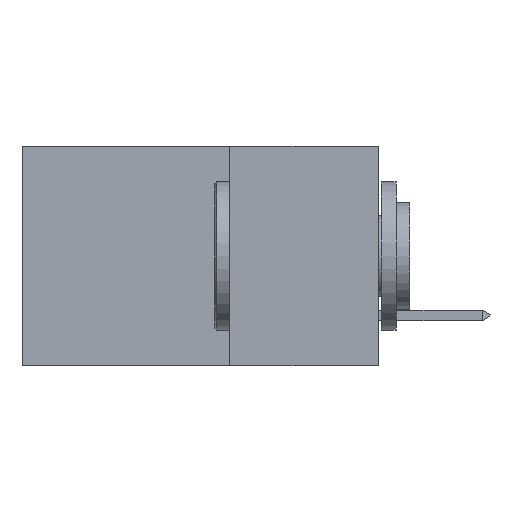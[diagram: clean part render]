
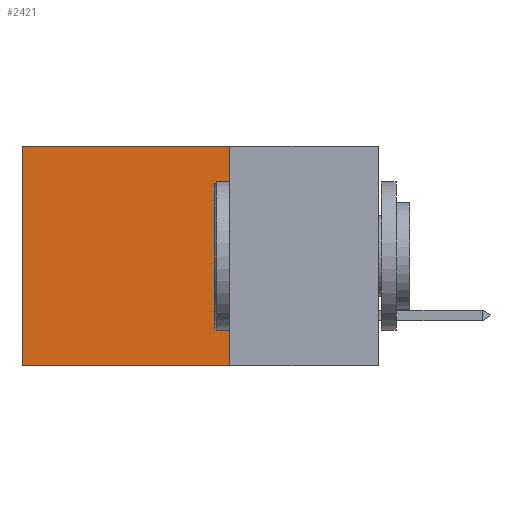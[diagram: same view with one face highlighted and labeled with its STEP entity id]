
A CAD part, left-side view. The second image highlights one B-rep face of the part: STEP entity #2421.
In plain terms, the highlighted planar face has unit normal (-1, 0, 0).
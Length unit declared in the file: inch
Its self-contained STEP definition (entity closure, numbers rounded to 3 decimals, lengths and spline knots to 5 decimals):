
#134 = CARTESIAN_POINT ( 'NONE',  ( 0.2615, 0.6, -0.37 ) ) ;
#1147 = VERTEX_POINT ( 'NONE', #4742 ) ;
#1373 = ORIENTED_EDGE ( 'NONE', *, *, #14383, .T. ) ;
#1987 = AXIS2_PLACEMENT_3D ( 'NONE', #10348, #13753, #13902 ) ;
#2421 = ADVANCED_FACE ( 'NONE', ( #10272 ), #9294, .F. ) ;
#2473 = EDGE_CURVE ( 'NONE', #3451, #9323, #14827, .T. ) ;
#2577 = CARTESIAN_POINT ( 'NONE',  ( 0.2615, 0.25, -0.37 ) ) ;
#2653 = LINE ( 'NONE', #2577, #9335 ) ;
#2990 = ORIENTED_EDGE ( 'NONE', *, *, #2473, .T. ) ;
#3451 = VERTEX_POINT ( 'NONE', #3565 ) ;
#3565 = CARTESIAN_POINT ( 'NONE',  ( 0.2615, 0.6, 0. ) ) ;
#4742 = CARTESIAN_POINT ( 'NONE',  ( 0.2615, 0.25, 0. ) ) ;
#4792 = DIRECTION ( 'NONE',  ( 0., 1., 0. ) ) ;
#5675 = CARTESIAN_POINT ( 'NONE',  ( 0.2615, 0.6, -0.37 ) ) ;
#5915 = LINE ( 'NONE', #13922, #9956 ) ;
#6710 = EDGE_LOOP ( 'NONE', ( #2990, #13027, #14347, #1373 ) ) ;
#6981 = LINE ( 'NONE', #12716, #7502 ) ;
#7502 = VECTOR ( 'NONE', #4792, 39.37008 ) ;
#7529 = VECTOR ( 'NONE', #12693, 39.37008 ) ;
#7780 = EDGE_CURVE ( 'NONE', #10533, #9323, #2653, .T. ) ;
#9294 = PLANE ( 'NONE',  #1987 ) ;
#9323 = VERTEX_POINT ( 'NONE', #134 ) ;
#9335 = VECTOR ( 'NONE', #10791, 39.37008 ) ;
#9956 = VECTOR ( 'NONE', #12791, 39.37008 ) ;
#10272 = FACE_OUTER_BOUND ( 'NONE', #6710, .T. ) ;
#10348 = CARTESIAN_POINT ( 'NONE',  ( 0.2615, 0.25, -0.37 ) ) ;
#10533 = VERTEX_POINT ( 'NONE', #10996 ) ;
#10791 = DIRECTION ( 'NONE',  ( 0., 1., 0. ) ) ;
#10996 = CARTESIAN_POINT ( 'NONE',  ( 0.2615, 0.25, -0.37 ) ) ;
#12693 = DIRECTION ( 'NONE',  ( 0., 0., -1. ) ) ;
#12716 = CARTESIAN_POINT ( 'NONE',  ( 0.2615, 0.25, 0. ) ) ;
#12791 = DIRECTION ( 'NONE',  ( 0., 0., -1. ) ) ;
#13027 = ORIENTED_EDGE ( 'NONE', *, *, #7780, .F. ) ;
#13753 = DIRECTION ( 'NONE',  ( 1., 0., 0. ) ) ;
#13902 = DIRECTION ( 'NONE',  ( 0., 0., -1. ) ) ;
#13922 = CARTESIAN_POINT ( 'NONE',  ( 0.2615, 0.25, -0.37 ) ) ;
#14347 = ORIENTED_EDGE ( 'NONE', *, *, #14433, .F. ) ;
#14383 = EDGE_CURVE ( 'NONE', #1147, #3451, #6981, .T. ) ;
#14433 = EDGE_CURVE ( 'NONE', #1147, #10533, #5915, .T. ) ;
#14827 = LINE ( 'NONE', #5675, #7529 ) ;
